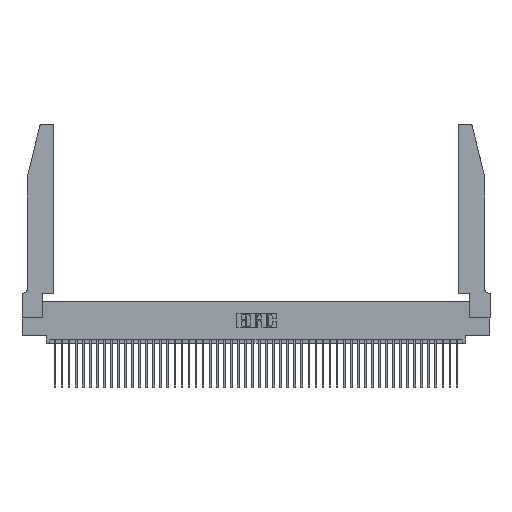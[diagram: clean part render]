
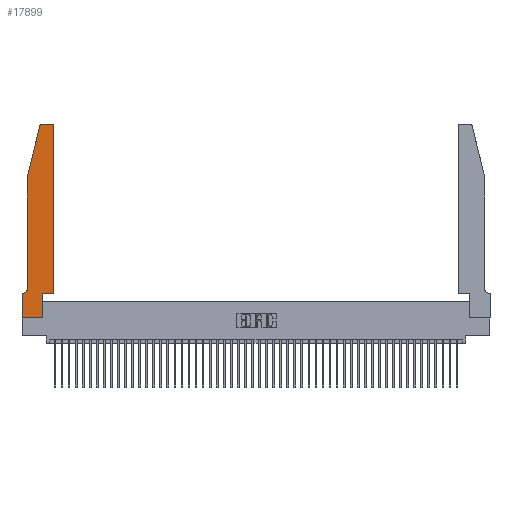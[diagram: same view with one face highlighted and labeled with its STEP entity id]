
A CAD part, top view. The second image highlights one B-rep face of the part: STEP entity #17899.
In plain terms, the highlighted planar face has unit normal (0, 0, 1).
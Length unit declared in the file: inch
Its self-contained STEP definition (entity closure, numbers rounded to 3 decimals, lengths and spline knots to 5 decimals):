
#320 = ORIENTED_EDGE ( 'NONE', *, *, #23090, .T. ) ;
#359 = CARTESIAN_POINT ( 'NONE',  ( 0.0055, 0.35, 0.37 ) ) ;
#537 = EDGE_CURVE ( 'NONE', #17906, #18026, #48011, .T. ) ;
#557 = LINE ( 'NONE', #10448, #20393 ) ;
#1000 = VERTEX_POINT ( 'NONE', #23902 ) ;
#1096 = LINE ( 'NONE', #20168, #14529 ) ;
#1416 = ORIENTED_EDGE ( 'NONE', *, *, #26702, .T. ) ;
#2098 = CARTESIAN_POINT ( 'NONE',  ( 0., 0., 0.37 ) ) ;
#2197 = DIRECTION ( 'NONE',  ( 1., 0., 0. ) ) ;
#3420 = VERTEX_POINT ( 'NONE', #14211 ) ;
#3571 = CARTESIAN_POINT ( 'NONE',  ( 0.0755, 0.35, 0.37 ) ) ;
#4225 = ORIENTED_EDGE ( 'NONE', *, *, #22114, .T. ) ;
#4585 = DIRECTION ( 'NONE',  ( 0., 0., 1. ) ) ;
#5817 = CARTESIAN_POINT ( 'NONE',  ( 0.284, 2.75, 0.37 ) ) ;
#6306 = DIRECTION ( 'NONE',  ( 0., -1., 0. ) ) ;
#6639 = ORIENTED_EDGE ( 'NONE', *, *, #15735, .T. ) ;
#8001 = ORIENTED_EDGE ( 'NONE', *, *, #24925, .T. ) ;
#8098 = CARTESIAN_POINT ( 'NONE',  ( 0.4505, 0.35, 0.37 ) ) ;
#8188 = DIRECTION ( 'NONE',  ( 1., 0., 0. ) ) ;
#8484 = VECTOR ( 'NONE', #6306, 39.37008 ) ;
#8522 = CARTESIAN_POINT ( 'NONE',  ( 0.2865, 0.35, 0.37 ) ) ;
#8616 = DIRECTION ( 'NONE',  ( -1., 0., 0. ) ) ;
#9528 = DIRECTION ( 'NONE',  ( 0., 0., 1. ) ) ;
#9585 = VECTOR ( 'NONE', #13524, 39.37008 ) ;
#10038 = DIRECTION ( 'NONE',  ( 0., 0., 1. ) ) ;
#10448 = CARTESIAN_POINT ( 'NONE',  ( 0.0755, 2., 0.37 ) ) ;
#11214 = AXIS2_PLACEMENT_3D ( 'NONE', #33767, #11412, #19058 ) ;
#11412 = DIRECTION ( 'NONE',  ( 0., 0., -1. ) ) ;
#11805 = VECTOR ( 'NONE', #12161, 39.37008 ) ;
#11960 = ORIENTED_EDGE ( 'NONE', *, *, #35464, .T. ) ;
#12131 = VERTEX_POINT ( 'NONE', #24375 ) ;
#12161 = DIRECTION ( 'NONE',  ( 1., 0., 0. ) ) ;
#12184 = EDGE_CURVE ( 'NONE', #12131, #19394, #24868, .T. ) ;
#13524 = DIRECTION ( 'NONE',  ( 0., -1., 0. ) ) ;
#13723 = DIRECTION ( 'NONE',  ( -0.239, -0.971, 0. ) ) ;
#13848 = CARTESIAN_POINT ( 'NONE',  ( 0., 0.35, 0.37 ) ) ;
#13929 = ORIENTED_EDGE ( 'NONE', *, *, #31130, .T. ) ;
#14211 = CARTESIAN_POINT ( 'NONE',  ( 0.2865, 0., 0.37 ) ) ;
#14529 = VECTOR ( 'NONE', #8616, 39.37008 ) ;
#14680 = EDGE_CURVE ( 'NONE', #18026, #31131, #47977, .T. ) ;
#15351 = AXIS2_PLACEMENT_3D ( 'NONE', #21114, #10038, #2197 ) ;
#15735 = EDGE_CURVE ( 'NONE', #24719, #1000, #43918, .T. ) ;
#16592 = AXIS2_PLACEMENT_3D ( 'NONE', #30875, #4585, #8188 ) ;
#16889 = CARTESIAN_POINT ( 'NONE',  ( 0.4505, 0.35, 0.37 ) ) ;
#17539 = CARTESIAN_POINT ( 'NONE',  ( 0.0755, 2., 0.37 ) ) ;
#17899 = ADVANCED_FACE ( 'NONE', ( #20358 ), #19425, .T. ) ;
#17906 = VERTEX_POINT ( 'NONE', #34275 ) ;
#18026 = VERTEX_POINT ( 'NONE', #359 ) ;
#19058 = DIRECTION ( 'NONE',  ( -1., 0., 0. ) ) ;
#19153 = LINE ( 'NONE', #8522, #42507 ) ;
#19394 = VERTEX_POINT ( 'NONE', #20599 ) ;
#19425 = PLANE ( 'NONE',  #16592 ) ;
#19659 = DIRECTION ( 'NONE',  ( 1., 0., 0. ) ) ;
#20168 = CARTESIAN_POINT ( 'NONE',  ( 0.2605, 2.75, 0.37 ) ) ;
#20358 = FACE_OUTER_BOUND ( 'NONE', #37957, .T. ) ;
#20393 = VECTOR ( 'NONE', #13723, 39.37008 ) ;
#20599 = CARTESIAN_POINT ( 'NONE',  ( 0.4205, 2.75, 0.37 ) ) ;
#21086 = DIRECTION ( 'NONE',  ( 1., 0., 0. ) ) ;
#21114 = CARTESIAN_POINT ( 'NONE',  ( 0.284, 2.72, 0.37 ) ) ;
#22114 = EDGE_CURVE ( 'NONE', #1000, #46969, #557, .T. ) ;
#23080 = AXIS2_PLACEMENT_3D ( 'NONE', #31871, #9528, #21086 ) ;
#23090 = EDGE_CURVE ( 'NONE', #38016, #3420, #41874, .T. ) ;
#23120 = ORIENTED_EDGE ( 'NONE', *, *, #41360, .T. ) ;
#23902 = CARTESIAN_POINT ( 'NONE',  ( 0.25487, 2.72718, 0.37 ) ) ;
#24375 = CARTESIAN_POINT ( 'NONE',  ( 0.4505, 2.72, 0.37 ) ) ;
#24719 = VERTEX_POINT ( 'NONE', #5817 ) ;
#24868 = CIRCLE ( 'NONE', #23080, 0.03 ) ;
#24925 = EDGE_CURVE ( 'NONE', #46969, #17906, #34171, .T. ) ;
#25039 = CARTESIAN_POINT ( 'NONE',  ( 0.4505, 0.35, 0.37 ) ) ;
#25269 = LINE ( 'NONE', #8098, #11805 ) ;
#25523 = CARTESIAN_POINT ( 'NONE',  ( 0.2865, 0.35, 0.37 ) ) ;
#26655 = DIRECTION ( 'NONE',  ( 0., 1., 0. ) ) ;
#26694 = ORIENTED_EDGE ( 'NONE', *, *, #12184, .T. ) ;
#26702 = EDGE_CURVE ( 'NONE', #43326, #36246, #25269, .T. ) ;
#30875 = CARTESIAN_POINT ( 'NONE',  ( 0., 0.35, 0.37 ) ) ;
#31130 = EDGE_CURVE ( 'NONE', #31131, #38016, #40535, .T. ) ;
#31131 = VERTEX_POINT ( 'NONE', #13848 ) ;
#31871 = CARTESIAN_POINT ( 'NONE',  ( 0.4205, 2.72, 0.37 ) ) ;
#33767 = CARTESIAN_POINT ( 'NONE',  ( 0.0055, 0.42, 0.37 ) ) ;
#34171 = LINE ( 'NONE', #17539, #8484 ) ;
#34275 = CARTESIAN_POINT ( 'NONE',  ( 0.0755, 0.42, 0.37 ) ) ;
#35464 = EDGE_CURVE ( 'NONE', #3420, #43326, #19153, .T. ) ;
#35832 = ORIENTED_EDGE ( 'NONE', *, *, #48085, .T. ) ;
#36246 = VERTEX_POINT ( 'NONE', #16889 ) ;
#37957 = EDGE_LOOP ( 'NONE', ( #35832, #6639, #4225, #8001, #39310, #44113, #13929, #320, #11960, #1416, #23120, #26694 ) ) ;
#38016 = VERTEX_POINT ( 'NONE', #46042 ) ;
#38685 = CARTESIAN_POINT ( 'NONE',  ( 0.0755, 2., 0.37 ) ) ;
#38729 = CARTESIAN_POINT ( 'NONE',  ( 0., 0., 0.37 ) ) ;
#39310 = ORIENTED_EDGE ( 'NONE', *, *, #537, .T. ) ;
#39506 = DIRECTION ( 'NONE',  ( 0., 1., 0. ) ) ;
#39796 = VECTOR ( 'NONE', #47908, 39.37008 ) ;
#40535 = LINE ( 'NONE', #2098, #9585 ) ;
#40707 = VECTOR ( 'NONE', #19659, 39.37008 ) ;
#41360 = EDGE_CURVE ( 'NONE', #36246, #12131, #45061, .T. ) ;
#41874 = LINE ( 'NONE', #38729, #40707 ) ;
#42507 = VECTOR ( 'NONE', #26655, 39.37008 ) ;
#43326 = VERTEX_POINT ( 'NONE', #25523 ) ;
#43918 = CIRCLE ( 'NONE', #15351, 0.03 ) ;
#44113 = ORIENTED_EDGE ( 'NONE', *, *, #14680, .T. ) ;
#44498 = VECTOR ( 'NONE', #39506, 39.37008 ) ;
#45061 = LINE ( 'NONE', #25039, #44498 ) ;
#46042 = CARTESIAN_POINT ( 'NONE',  ( 0., 0., 0.37 ) ) ;
#46969 = VERTEX_POINT ( 'NONE', #38685 ) ;
#47908 = DIRECTION ( 'NONE',  ( -1., 0., 0. ) ) ;
#47977 = LINE ( 'NONE', #3571, #39796 ) ;
#48011 = CIRCLE ( 'NONE', #11214, 0.07 ) ;
#48085 = EDGE_CURVE ( 'NONE', #19394, #24719, #1096, .T. ) ;
